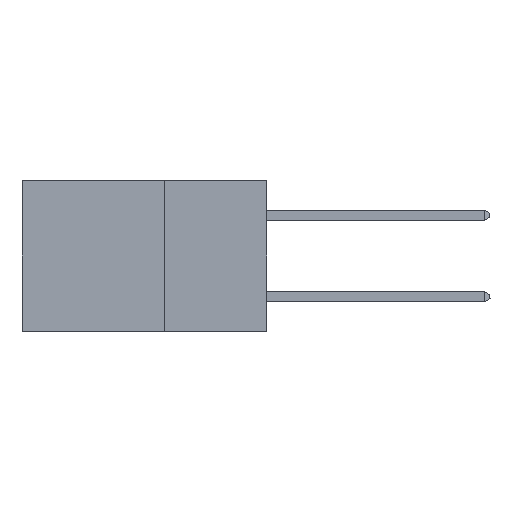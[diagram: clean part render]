
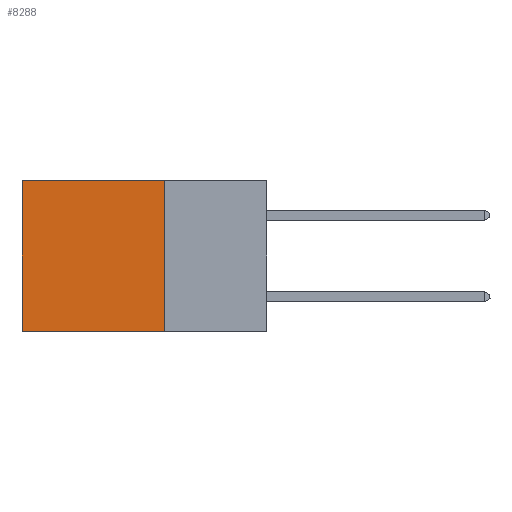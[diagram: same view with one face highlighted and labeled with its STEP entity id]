
A CAD part, left-side view. The second image highlights one B-rep face of the part: STEP entity #8288.
In plain terms, the highlighted planar face has unit normal (-1, 0, 0).
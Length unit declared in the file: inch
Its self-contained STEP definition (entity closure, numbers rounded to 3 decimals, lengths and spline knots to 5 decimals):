
#76 = CARTESIAN_POINT ( 'NONE',  ( 0.2875, 0.25, 0. ) ) ;
#227 = DIRECTION ( 'NONE',  ( 0., 0., -1. ) ) ;
#1087 = PLANE ( 'NONE',  #14242 ) ;
#1261 = FACE_OUTER_BOUND ( 'NONE', #2528, .T. ) ;
#2018 = ORIENTED_EDGE ( 'NONE', *, *, #3233, .T. ) ;
#2312 = DIRECTION ( 'NONE',  ( 0., 0., -1. ) ) ;
#2434 = DIRECTION ( 'NONE',  ( 0., 1., 0. ) ) ;
#2509 = ORIENTED_EDGE ( 'NONE', *, *, #9776, .F. ) ;
#2528 = EDGE_LOOP ( 'NONE', ( #11237, #2509, #10770, #2018 ) ) ;
#3233 = EDGE_CURVE ( 'NONE', #6719, #8897, #11549, .T. ) ;
#3271 = LINE ( 'NONE', #76, #6988 ) ;
#5088 = LINE ( 'NONE', #13808, #13410 ) ;
#5439 = CARTESIAN_POINT ( 'NONE',  ( 0.2875, 0.25, -0.37 ) ) ;
#6214 = VECTOR ( 'NONE', #2434, 39.37008 ) ;
#6489 = CARTESIAN_POINT ( 'NONE',  ( 0.2875, 0.6, 0. ) ) ;
#6719 = VERTEX_POINT ( 'NONE', #8591 ) ;
#6988 = VECTOR ( 'NONE', #227, 39.37008 ) ;
#7317 = CARTESIAN_POINT ( 'NONE',  ( 0.2875, 0.25, 0. ) ) ;
#8288 = ADVANCED_FACE ( 'NONE', ( #1261 ), #1087, .F. ) ;
#8591 = CARTESIAN_POINT ( 'NONE',  ( 0.2875, 0.25, 0. ) ) ;
#8670 = EDGE_CURVE ( 'NONE', #6719, #14206, #3271, .T. ) ;
#8897 = VERTEX_POINT ( 'NONE', #6489 ) ;
#9776 = EDGE_CURVE ( 'NONE', #14206, #15067, #5088, .T. ) ;
#10770 = ORIENTED_EDGE ( 'NONE', *, *, #8670, .F. ) ;
#10786 = VECTOR ( 'NONE', #2312, 39.37008 ) ;
#11237 = ORIENTED_EDGE ( 'NONE', *, *, #14981, .T. ) ;
#11255 = CARTESIAN_POINT ( 'NONE',  ( 0.2875, 0.6, -0.37 ) ) ;
#11549 = LINE ( 'NONE', #13028, #6214 ) ;
#11724 = LINE ( 'NONE', #12813, #10786 ) ;
#11930 = DIRECTION ( 'NONE',  ( 0., 0., -1. ) ) ;
#12699 = DIRECTION ( 'NONE',  ( 0., 1., 0. ) ) ;
#12813 = CARTESIAN_POINT ( 'NONE',  ( 0.2875, 0.6, 0. ) ) ;
#13028 = CARTESIAN_POINT ( 'NONE',  ( 0.2875, 0.25, 0. ) ) ;
#13410 = VECTOR ( 'NONE', #12699, 39.37008 ) ;
#13808 = CARTESIAN_POINT ( 'NONE',  ( 0.2875, 0.25, -0.37 ) ) ;
#14206 = VERTEX_POINT ( 'NONE', #5439 ) ;
#14242 = AXIS2_PLACEMENT_3D ( 'NONE', #7317, #14274, #11930 ) ;
#14274 = DIRECTION ( 'NONE',  ( 1., 0., 0. ) ) ;
#14981 = EDGE_CURVE ( 'NONE', #8897, #15067, #11724, .T. ) ;
#15067 = VERTEX_POINT ( 'NONE', #11255 ) ;
